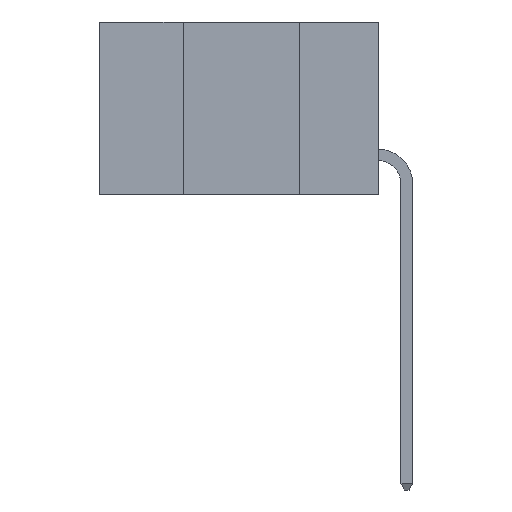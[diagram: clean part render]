
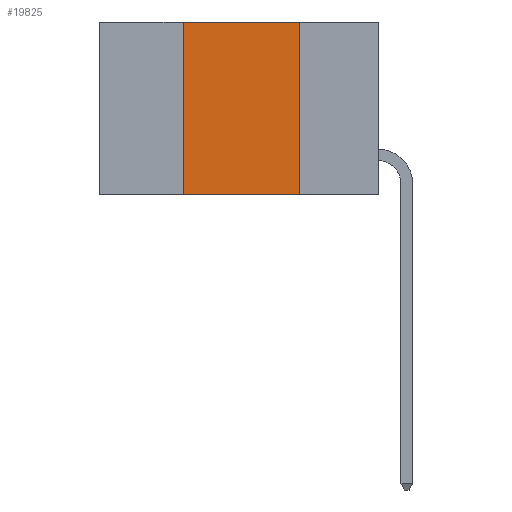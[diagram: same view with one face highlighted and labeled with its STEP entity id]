
A CAD part, left-side view. The second image highlights one B-rep face of the part: STEP entity #19825.
In plain terms, the highlighted planar face has unit normal (-1, 0, 0).
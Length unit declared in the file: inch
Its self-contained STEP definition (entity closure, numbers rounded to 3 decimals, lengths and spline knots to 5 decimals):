
#104 = ORIENTED_EDGE ( 'NONE', *, *, #5081, .F. ) ;
#178 = EDGE_CURVE ( 'NONE', #9064, #12081, #15179, .T. ) ;
#249 = DIRECTION ( 'NONE',  ( 0., -1., 0. ) ) ;
#353 = VECTOR ( 'NONE', #249, 39.37008 ) ;
#1009 = CARTESIAN_POINT ( 'NONE',  ( 0., 0.42, 0. ) ) ;
#1584 = DIRECTION ( 'NONE',  ( 1., 0., 0. ) ) ;
#1623 = CARTESIAN_POINT ( 'NONE',  ( 0., 0.42, -0.37 ) ) ;
#1694 = EDGE_CURVE ( 'NONE', #19441, #14406, #9396, .T. ) ;
#1957 = VECTOR ( 'NONE', #2986, 39.37008 ) ;
#2071 = ORIENTED_EDGE ( 'NONE', *, *, #1694, .F. ) ;
#2986 = DIRECTION ( 'NONE',  ( 0., 0., 1. ) ) ;
#3485 = CARTESIAN_POINT ( 'NONE',  ( 0., 0.6, -0.37 ) ) ;
#3992 = ORIENTED_EDGE ( 'NONE', *, *, #178, .F. ) ;
#4136 = CARTESIAN_POINT ( 'NONE',  ( 0., 0.42, -0.37 ) ) ;
#5081 = EDGE_CURVE ( 'NONE', #12081, #19441, #5334, .T. ) ;
#5334 = LINE ( 'NONE', #16551, #19327 ) ;
#7185 = CARTESIAN_POINT ( 'NONE',  ( 0., 0.17, 0. ) ) ;
#9064 = VERTEX_POINT ( 'NONE', #1623 ) ;
#9396 = LINE ( 'NONE', #20170, #18004 ) ;
#9767 = LINE ( 'NONE', #3485, #353 ) ;
#11609 = PLANE ( 'NONE',  #17432 ) ;
#12081 = VERTEX_POINT ( 'NONE', #1009 ) ;
#12475 = EDGE_CURVE ( 'NONE', #9064, #14406, #9767, .T. ) ;
#13233 = DIRECTION ( 'NONE',  ( 0., 0., -1. ) ) ;
#13708 = DIRECTION ( 'NONE',  ( 0., 0., -1. ) ) ;
#14071 = ORIENTED_EDGE ( 'NONE', *, *, #12475, .T. ) ;
#14406 = VERTEX_POINT ( 'NONE', #19758 ) ;
#15179 = LINE ( 'NONE', #4136, #1957 ) ;
#16496 = DIRECTION ( 'NONE',  ( 0., -1., 0. ) ) ;
#16551 = CARTESIAN_POINT ( 'NONE',  ( 0., 0.6, 0. ) ) ;
#17432 = AXIS2_PLACEMENT_3D ( 'NONE', #19558, #1584, #13233 ) ;
#18004 = VECTOR ( 'NONE', #13708, 39.37008 ) ;
#18173 = FACE_OUTER_BOUND ( 'NONE', #18563, .T. ) ;
#18563 = EDGE_LOOP ( 'NONE', ( #2071, #104, #3992, #14071 ) ) ;
#19327 = VECTOR ( 'NONE', #16496, 39.37008 ) ;
#19441 = VERTEX_POINT ( 'NONE', #7185 ) ;
#19558 = CARTESIAN_POINT ( 'NONE',  ( 0., 0.6, 0. ) ) ;
#19758 = CARTESIAN_POINT ( 'NONE',  ( 0., 0.17, -0.37 ) ) ;
#19825 = ADVANCED_FACE ( 'NONE', ( #18173 ), #11609, .F. ) ;
#20170 = CARTESIAN_POINT ( 'NONE',  ( 0., 0.17, -0.37 ) ) ;
